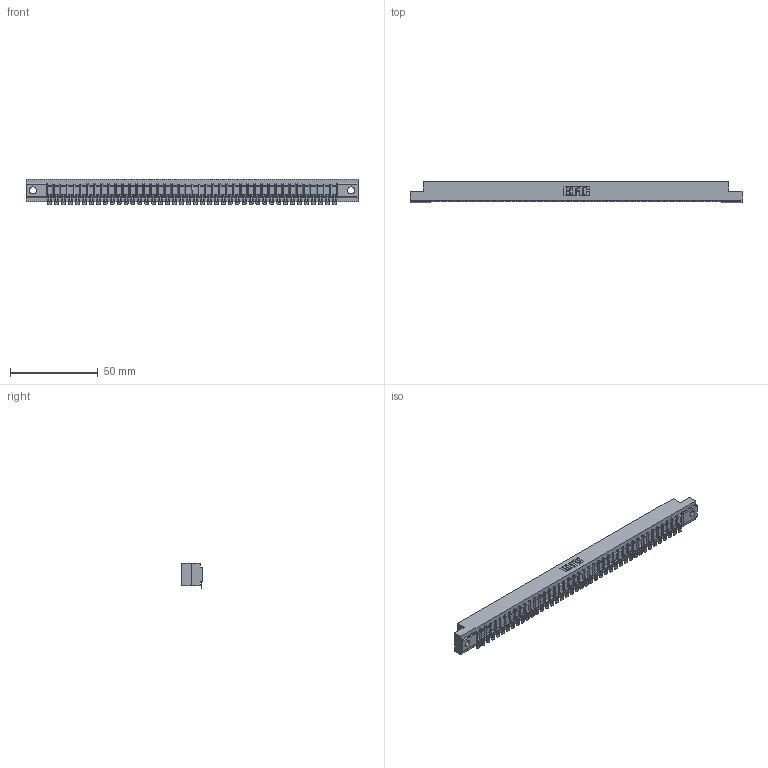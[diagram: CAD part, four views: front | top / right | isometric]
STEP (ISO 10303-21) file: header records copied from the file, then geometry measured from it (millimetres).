
FILE_DESCRIPTION (( 'STEP AP203' ), '1' );
FILE_NAME ('357-042-454-104.STEP', '2020-10-03T11:15:09', ( '' ), ( '' ), 'SwSTEP 2.0', 'SolidWorks 2020', '' );
FILE_SCHEMA (( 'CONFIG_CONTROL_DESIGN' ));
Length unit declared in the file: inch
Products named in the file (3): 357-042-454-104; 307 Part_.156 Dia Mounting Holes; 307-290-002_554
Assembly tree (43 placements, depth 2):
  357-042-454-104
    307 Part_.156 Dia Mounting Holes
    307-290-002_554  x42
Bounding box: 189.43 x 12.01 x 14.52 mm (x, y, z)
Volume: 20180.9 mm3; surface area: 25372.2 mm2
Topology: 43 solids, 43 shells, 3577 faces, 10985 edges, 7206 vertices
Faces by surface type: plane 2016, cylinder 1475, sphere 86
Entity records: 37389 total; most frequent: CARTESIAN_POINT 6312, ORIENTED_EDGE 6300, DIRECTION 6130, EDGE_CURVE 3150, LINE 2414, VECTOR 2414, VERTEX_POINT 2040, AXIS2_PLACEMENT_3D 1858
